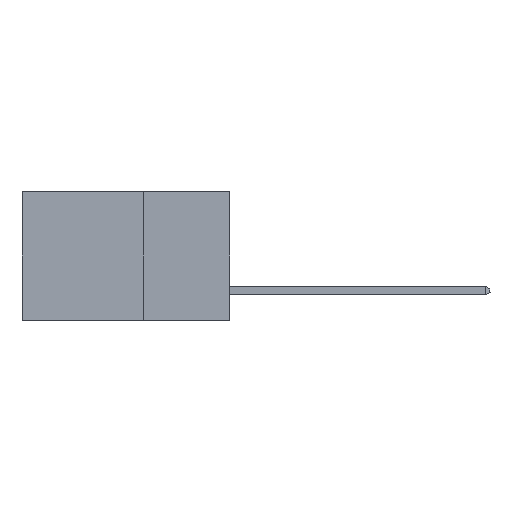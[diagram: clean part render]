
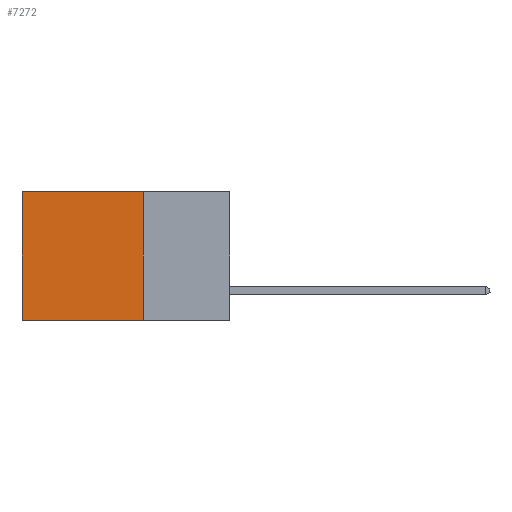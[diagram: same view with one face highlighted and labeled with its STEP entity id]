
A CAD part, left-side view. The second image highlights one B-rep face of the part: STEP entity #7272.
In plain terms, the highlighted planar face has unit normal (-1, 0, 0).
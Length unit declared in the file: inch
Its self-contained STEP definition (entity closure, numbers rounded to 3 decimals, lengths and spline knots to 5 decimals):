
#160 = CARTESIAN_POINT ( 'NONE',  ( 0.298, 0.6, 0. ) ) ;
#769 = CARTESIAN_POINT ( 'NONE',  ( 0.298, 0.25, 0. ) ) ;
#844 = VECTOR ( 'NONE', #888, 39.37008 ) ;
#888 = DIRECTION ( 'NONE',  ( 0., 0., -1. ) ) ;
#1639 = EDGE_CURVE ( 'NONE', #8320, #10346, #2045, .T. ) ;
#1804 = LINE ( 'NONE', #8277, #11238 ) ;
#2045 = LINE ( 'NONE', #12346, #6414 ) ;
#2808 = AXIS2_PLACEMENT_3D ( 'NONE', #769, #6675, #9576 ) ;
#2971 = EDGE_CURVE ( 'NONE', #6642, #6720, #1804, .T. ) ;
#3573 = EDGE_LOOP ( 'NONE', ( #11711, #4668, #5562, #7469 ) ) ;
#3932 = EDGE_CURVE ( 'NONE', #8320, #6642, #4427, .T. ) ;
#4427 = LINE ( 'NONE', #5687, #844 ) ;
#4668 = ORIENTED_EDGE ( 'NONE', *, *, #2971, .F. ) ;
#5562 = ORIENTED_EDGE ( 'NONE', *, *, #3932, .F. ) ;
#5687 = CARTESIAN_POINT ( 'NONE',  ( 0.298, 0.25, 0. ) ) ;
#6414 = VECTOR ( 'NONE', #9315, 39.37008 ) ;
#6642 = VERTEX_POINT ( 'NONE', #12701 ) ;
#6675 = DIRECTION ( 'NONE',  ( 1., 0., 0. ) ) ;
#6720 = VERTEX_POINT ( 'NONE', #6851 ) ;
#6851 = CARTESIAN_POINT ( 'NONE',  ( 0.298, 0.6, -0.37 ) ) ;
#6982 = FACE_OUTER_BOUND ( 'NONE', #3573, .T. ) ;
#7272 = ADVANCED_FACE ( 'NONE', ( #6982 ), #10468, .F. ) ;
#7469 = ORIENTED_EDGE ( 'NONE', *, *, #1639, .T. ) ;
#7975 = CARTESIAN_POINT ( 'NONE',  ( 0.298, 0.6, 0. ) ) ;
#8277 = CARTESIAN_POINT ( 'NONE',  ( 0.298, 0.25, -0.37 ) ) ;
#8320 = VERTEX_POINT ( 'NONE', #12499 ) ;
#9106 = EDGE_CURVE ( 'NONE', #10346, #6720, #12775, .T. ) ;
#9273 = DIRECTION ( 'NONE',  ( 0., 1., 0. ) ) ;
#9315 = DIRECTION ( 'NONE',  ( 0., 1., 0. ) ) ;
#9576 = DIRECTION ( 'NONE',  ( 0., 0., -1. ) ) ;
#10346 = VERTEX_POINT ( 'NONE', #7975 ) ;
#10468 = PLANE ( 'NONE',  #2808 ) ;
#10626 = VECTOR ( 'NONE', #11100, 39.37008 ) ;
#11100 = DIRECTION ( 'NONE',  ( 0., 0., -1. ) ) ;
#11238 = VECTOR ( 'NONE', #9273, 39.37008 ) ;
#11711 = ORIENTED_EDGE ( 'NONE', *, *, #9106, .T. ) ;
#12346 = CARTESIAN_POINT ( 'NONE',  ( 0.298, 0.25, 0. ) ) ;
#12499 = CARTESIAN_POINT ( 'NONE',  ( 0.298, 0.25, 0. ) ) ;
#12701 = CARTESIAN_POINT ( 'NONE',  ( 0.298, 0.25, -0.37 ) ) ;
#12775 = LINE ( 'NONE', #160, #10626 ) ;
